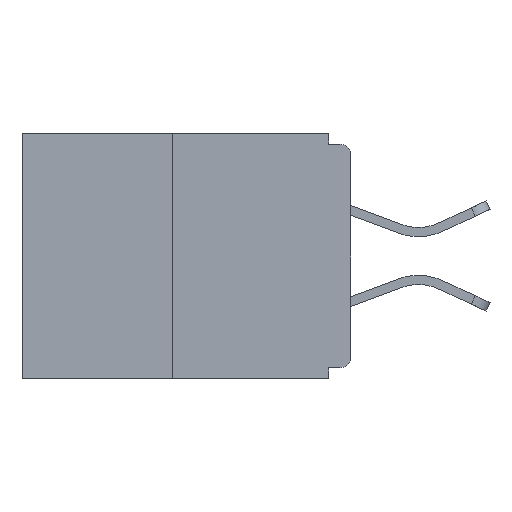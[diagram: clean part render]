
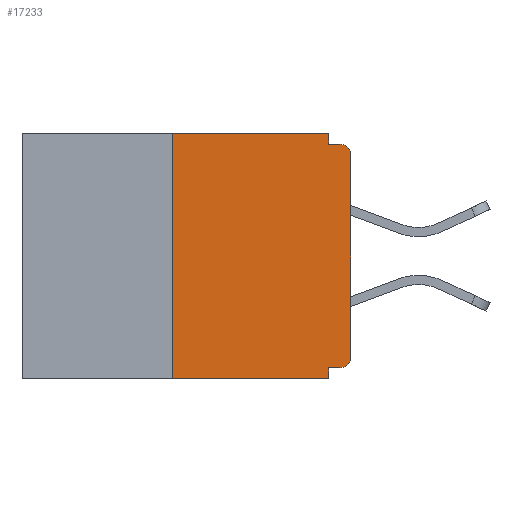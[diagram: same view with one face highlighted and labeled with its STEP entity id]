
A CAD part, left-side view. The second image highlights one B-rep face of the part: STEP entity #17233.
In plain terms, the highlighted planar face has unit normal (-1, 0, 0).
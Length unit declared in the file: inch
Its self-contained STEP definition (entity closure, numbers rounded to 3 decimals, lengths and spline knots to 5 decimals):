
#16 = CARTESIAN_POINT ( 'NONE',  ( 0., 0.031, 0. ) ) ;
#20 = ORIENTED_EDGE ( 'NONE', *, *, #5015, .F. ) ;
#333 = EDGE_CURVE ( 'NONE', #16756, #995, #2001, .T. ) ;
#581 = VECTOR ( 'NONE', #4347, 39.37008 ) ;
#601 = DIRECTION ( 'NONE',  ( 0., 0., -1. ) ) ;
#892 = ORIENTED_EDGE ( 'NONE', *, *, #18138, .F. ) ;
#987 = CARTESIAN_POINT ( 'NONE',  ( 0., 0., -0.328 ) ) ;
#995 = VERTEX_POINT ( 'NONE', #14758 ) ;
#1176 = LINE ( 'NONE', #987, #6110 ) ;
#1207 = CARTESIAN_POINT ( 'NONE',  ( 0., 0.015, -0.03 ) ) ;
#1414 = CARTESIAN_POINT ( 'NONE',  ( 0., 0., -0.015 ) ) ;
#1662 = VECTOR ( 'NONE', #7055, 39.37008 ) ;
#1846 = AXIS2_PLACEMENT_3D ( 'NONE', #17296, #16841, #12262 ) ;
#2001 = LINE ( 'NONE', #16994, #10303 ) ;
#2006 = EDGE_CURVE ( 'NONE', #3844, #9433, #13314, .T. ) ;
#2201 = EDGE_CURVE ( 'NONE', #6143, #7601, #9219, .T. ) ;
#2271 = ORIENTED_EDGE ( 'NONE', *, *, #12034, .T. ) ;
#2879 = VERTEX_POINT ( 'NONE', #4731 ) ;
#3228 = DIRECTION ( 'NONE',  ( -1., 0., 0. ) ) ;
#3585 = ORIENTED_EDGE ( 'NONE', *, *, #7161, .T. ) ;
#3749 = CARTESIAN_POINT ( 'NONE',  ( 0., 0.015, -0.015 ) ) ;
#3844 = VERTEX_POINT ( 'NONE', #13493 ) ;
#4006 = VECTOR ( 'NONE', #10610, 39.37008 ) ;
#4347 = DIRECTION ( 'NONE',  ( 0., -1., 0. ) ) ;
#4696 = DIRECTION ( 'NONE',  ( 0., 0., -1. ) ) ;
#4731 = CARTESIAN_POINT ( 'NONE',  ( 0., 0., -0.313 ) ) ;
#5015 = EDGE_CURVE ( 'NONE', #5073, #6143, #15298, .T. ) ;
#5056 = LINE ( 'NONE', #9542, #15833 ) ;
#5060 = EDGE_CURVE ( 'NONE', #7601, #3844, #5056, .T. ) ;
#5073 = VERTEX_POINT ( 'NONE', #5429 ) ;
#5166 = AXIS2_PLACEMENT_3D ( 'NONE', #18126, #3228, #4696 ) ;
#5429 = CARTESIAN_POINT ( 'NONE',  ( 0., 0.25, -0.343 ) ) ;
#6093 = DIRECTION ( 'NONE',  ( 0., -1., 0. ) ) ;
#6110 = VECTOR ( 'NONE', #17526, 39.37008 ) ;
#6143 = VERTEX_POINT ( 'NONE', #11606 ) ;
#6196 = ORIENTED_EDGE ( 'NONE', *, *, #5060, .F. ) ;
#6261 = EDGE_CURVE ( 'NONE', #15590, #2879, #9529, .T. ) ;
#6492 = CARTESIAN_POINT ( 'NONE',  ( 0., 0.031, -0.328 ) ) ;
#6962 = FACE_OUTER_BOUND ( 'NONE', #10506, .T. ) ;
#7055 = DIRECTION ( 'NONE',  ( 0., 0., 1. ) ) ;
#7161 = EDGE_CURVE ( 'NONE', #7267, #9433, #13441, .T. ) ;
#7267 = VERTEX_POINT ( 'NONE', #15423 ) ;
#7318 = DIRECTION ( 'NONE',  ( -1., 0., 0. ) ) ;
#7601 = VERTEX_POINT ( 'NONE', #16 ) ;
#8797 = ORIENTED_EDGE ( 'NONE', *, *, #2201, .F. ) ;
#9219 = LINE ( 'NONE', #15064, #12387 ) ;
#9279 = ORIENTED_EDGE ( 'NONE', *, *, #12828, .T. ) ;
#9433 = VERTEX_POINT ( 'NONE', #3749 ) ;
#9529 = CIRCLE ( 'NONE', #5166, 0.015 ) ;
#9542 = CARTESIAN_POINT ( 'NONE',  ( 0., 0.031, 0. ) ) ;
#10016 = AXIS2_PLACEMENT_3D ( 'NONE', #1207, #7318, #19097 ) ;
#10303 = VECTOR ( 'NONE', #12321, 39.37008 ) ;
#10506 = EDGE_LOOP ( 'NONE', ( #8797, #20, #2271, #14051, #892, #17888, #9279, #3585, #15826, #6196 ) ) ;
#10610 = DIRECTION ( 'NONE',  ( 0., 0., 1. ) ) ;
#11606 = CARTESIAN_POINT ( 'NONE',  ( 0., 0.25, 0. ) ) ;
#11673 = CARTESIAN_POINT ( 'NONE',  ( 0., 0.46, -0.343 ) ) ;
#11732 = LINE ( 'NONE', #16125, #1662 ) ;
#12034 = EDGE_CURVE ( 'NONE', #5073, #995, #13046, .T. ) ;
#12087 = CARTESIAN_POINT ( 'NONE',  ( 0., 0.25, 0. ) ) ;
#12262 = DIRECTION ( 'NONE',  ( 0., 0., -1. ) ) ;
#12321 = DIRECTION ( 'NONE',  ( 0., 0., -1. ) ) ;
#12387 = VECTOR ( 'NONE', #6093, 39.37008 ) ;
#12828 = EDGE_CURVE ( 'NONE', #2879, #7267, #11732, .T. ) ;
#13046 = LINE ( 'NONE', #11673, #13141 ) ;
#13141 = VECTOR ( 'NONE', #15090, 39.37008 ) ;
#13314 = LINE ( 'NONE', #1414, #581 ) ;
#13441 = CIRCLE ( 'NONE', #10016, 0.015 ) ;
#13493 = CARTESIAN_POINT ( 'NONE',  ( 0., 0.031, -0.015 ) ) ;
#13610 = CARTESIAN_POINT ( 'NONE',  ( 0., 0.015, -0.328 ) ) ;
#14051 = ORIENTED_EDGE ( 'NONE', *, *, #333, .F. ) ;
#14758 = CARTESIAN_POINT ( 'NONE',  ( 0., 0.031, -0.343 ) ) ;
#15064 = CARTESIAN_POINT ( 'NONE',  ( 0., 0.46, 0. ) ) ;
#15090 = DIRECTION ( 'NONE',  ( 0., -1., 0. ) ) ;
#15298 = LINE ( 'NONE', #12087, #4006 ) ;
#15423 = CARTESIAN_POINT ( 'NONE',  ( 0., 0., -0.03 ) ) ;
#15590 = VERTEX_POINT ( 'NONE', #13610 ) ;
#15749 = PLANE ( 'NONE',  #1846 ) ;
#15826 = ORIENTED_EDGE ( 'NONE', *, *, #2006, .F. ) ;
#15833 = VECTOR ( 'NONE', #601, 39.37008 ) ;
#16125 = CARTESIAN_POINT ( 'NONE',  ( 0., 0., 0. ) ) ;
#16756 = VERTEX_POINT ( 'NONE', #6492 ) ;
#16841 = DIRECTION ( 'NONE',  ( 1., 0., 0. ) ) ;
#16994 = CARTESIAN_POINT ( 'NONE',  ( 0., 0.031, -0.343 ) ) ;
#17233 = ADVANCED_FACE ( 'NONE', ( #6962 ), #15749, .F. ) ;
#17296 = CARTESIAN_POINT ( 'NONE',  ( 0., 0.46, 0. ) ) ;
#17526 = DIRECTION ( 'NONE',  ( 0., 1., 0. ) ) ;
#17888 = ORIENTED_EDGE ( 'NONE', *, *, #6261, .T. ) ;
#18126 = CARTESIAN_POINT ( 'NONE',  ( 0., 0.015, -0.313 ) ) ;
#18138 = EDGE_CURVE ( 'NONE', #15590, #16756, #1176, .T. ) ;
#19097 = DIRECTION ( 'NONE',  ( 0., 0., -1. ) ) ;
